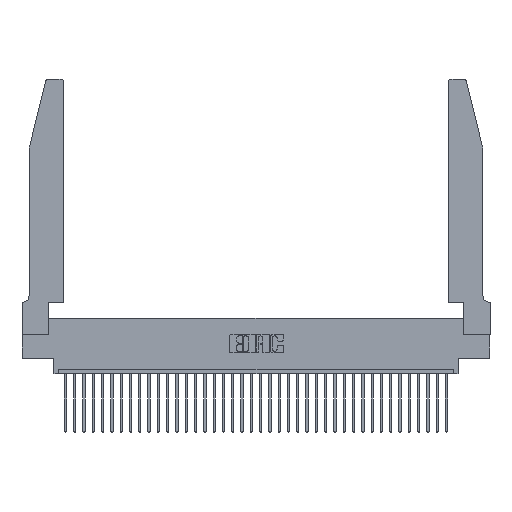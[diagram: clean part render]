
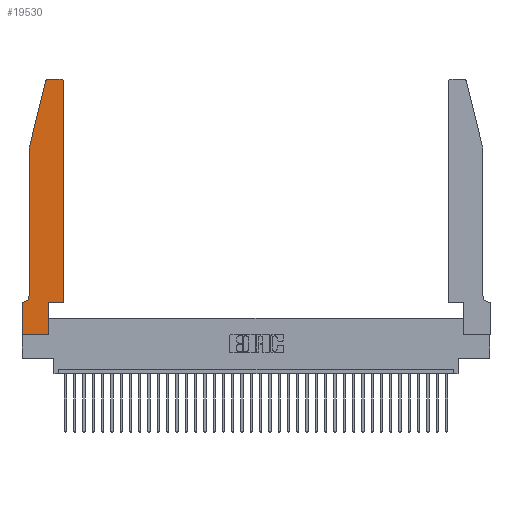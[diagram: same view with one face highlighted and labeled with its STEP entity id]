
A CAD part, top view. The second image highlights one B-rep face of the part: STEP entity #19530.
In plain terms, the highlighted planar face has unit normal (0, 0, 1).
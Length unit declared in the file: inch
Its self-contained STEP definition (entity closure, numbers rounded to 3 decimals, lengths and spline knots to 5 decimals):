
#104 = ORIENTED_EDGE ( 'NONE', *, *, #18381, .T. ) ;
#1021 = ORIENTED_EDGE ( 'NONE', *, *, #34340, .T. ) ;
#1047 = DIRECTION ( 'NONE',  ( 0., 0., 1. ) ) ;
#1149 = EDGE_CURVE ( 'NONE', #9233, #17301, #22306, .T. ) ;
#1381 = LINE ( 'NONE', #8915, #28766 ) ;
#1990 = DIRECTION ( 'NONE',  ( 0., 0., -1. ) ) ;
#2194 = DIRECTION ( 'NONE',  ( 0., -1., 0. ) ) ;
#2860 = CARTESIAN_POINT ( 'NONE',  ( 0.2865, 0.35, 0.37 ) ) ;
#3913 = CARTESIAN_POINT ( 'NONE',  ( 0.0755, 2., 0.37 ) ) ;
#4908 = ORIENTED_EDGE ( 'NONE', *, *, #8426, .T. ) ;
#5167 = CARTESIAN_POINT ( 'NONE',  ( 0.4505, 0.35, 0.37 ) ) ;
#5581 = VERTEX_POINT ( 'NONE', #16289 ) ;
#5893 = LINE ( 'NONE', #32503, #34131 ) ;
#6058 = ORIENTED_EDGE ( 'NONE', *, *, #6777, .T. ) ;
#6255 = PLANE ( 'NONE',  #33930 ) ;
#6259 = CARTESIAN_POINT ( 'NONE',  ( 0.4205, 2.75, 0.37 ) ) ;
#6381 = DIRECTION ( 'NONE',  ( 1., 0., 0. ) ) ;
#6386 = VECTOR ( 'NONE', #28680, 39.37008 ) ;
#6445 = CARTESIAN_POINT ( 'NONE',  ( 0.4505, 2.72, 0.37 ) ) ;
#6777 = EDGE_CURVE ( 'NONE', #31372, #21682, #1381, .T. ) ;
#7973 = DIRECTION ( 'NONE',  ( 0., 1., 0. ) ) ;
#8138 = CARTESIAN_POINT ( 'NONE',  ( 0.2865, 0., 0.37 ) ) ;
#8152 = FACE_OUTER_BOUND ( 'NONE', #36357, .T. ) ;
#8426 = EDGE_CURVE ( 'NONE', #9585, #5581, #9651, .T. ) ;
#8915 = CARTESIAN_POINT ( 'NONE',  ( 0.0755, 0.35, 0.37 ) ) ;
#9003 = VECTOR ( 'NONE', #2194, 39.37008 ) ;
#9174 = DIRECTION ( 'NONE',  ( -1., 0., 0. ) ) ;
#9233 = VERTEX_POINT ( 'NONE', #18907 ) ;
#9259 = ORIENTED_EDGE ( 'NONE', *, *, #11020, .T. ) ;
#9376 = DIRECTION ( 'NONE',  ( -1., 0., 0. ) ) ;
#9585 = VERTEX_POINT ( 'NONE', #6259 ) ;
#9651 = LINE ( 'NONE', #29414, #15865 ) ;
#9731 = VERTEX_POINT ( 'NONE', #2860 ) ;
#9755 = VERTEX_POINT ( 'NONE', #19752 ) ;
#10150 = DIRECTION ( 'NONE',  ( 1., 0., 0. ) ) ;
#10426 = ORIENTED_EDGE ( 'NONE', *, *, #25090, .T. ) ;
#11020 = EDGE_CURVE ( 'NONE', #18442, #15830, #34611, .T. ) ;
#11919 = DIRECTION ( 'NONE',  ( 0., 0., 1. ) ) ;
#12272 = VERTEX_POINT ( 'NONE', #26230 ) ;
#12887 = DIRECTION ( 'NONE',  ( 0., 0., 1. ) ) ;
#13012 = CARTESIAN_POINT ( 'NONE',  ( 0.4205, 2.72, 0.37 ) ) ;
#13457 = CARTESIAN_POINT ( 'NONE',  ( 0., 0., 0.37 ) ) ;
#13645 = CIRCLE ( 'NONE', #14404, 0.07 ) ;
#14021 = CARTESIAN_POINT ( 'NONE',  ( 0., 0., 0.37 ) ) ;
#14402 = CARTESIAN_POINT ( 'NONE',  ( 0., 0.35, 0.37 ) ) ;
#14404 = AXIS2_PLACEMENT_3D ( 'NONE', #25024, #1990, #27803 ) ;
#14706 = AXIS2_PLACEMENT_3D ( 'NONE', #29063, #1047, #32008 ) ;
#15378 = CARTESIAN_POINT ( 'NONE',  ( 0.0755, 0.42, 0.37 ) ) ;
#15453 = DIRECTION ( 'NONE',  ( 1., 0., 0. ) ) ;
#15830 = VERTEX_POINT ( 'NONE', #6445 ) ;
#15865 = VECTOR ( 'NONE', #9376, 39.37008 ) ;
#16289 = CARTESIAN_POINT ( 'NONE',  ( 0.284, 2.75, 0.37 ) ) ;
#16470 = VECTOR ( 'NONE', #27167, 39.37008 ) ;
#16622 = LINE ( 'NONE', #33528, #21451 ) ;
#16752 = ORIENTED_EDGE ( 'NONE', *, *, #1149, .T. ) ;
#16929 = VERTEX_POINT ( 'NONE', #8138 ) ;
#17301 = VERTEX_POINT ( 'NONE', #15378 ) ;
#18087 = EDGE_CURVE ( 'NONE', #21682, #12272, #34249, .T. ) ;
#18208 = ORIENTED_EDGE ( 'NONE', *, *, #24212, .T. ) ;
#18381 = EDGE_CURVE ( 'NONE', #5581, #9755, #33886, .T. ) ;
#18442 = VERTEX_POINT ( 'NONE', #23598 ) ;
#18907 = CARTESIAN_POINT ( 'NONE',  ( 0.0755, 2., 0.37 ) ) ;
#19153 = ORIENTED_EDGE ( 'NONE', *, *, #18087, .T. ) ;
#19207 = ORIENTED_EDGE ( 'NONE', *, *, #26116, .T. ) ;
#19271 = VECTOR ( 'NONE', #22269, 39.37008 ) ;
#19530 = ADVANCED_FACE ( 'NONE', ( #8152 ), #6255, .T. ) ;
#19752 = CARTESIAN_POINT ( 'NONE',  ( 0.25487, 2.72718, 0.37 ) ) ;
#20029 = DIRECTION ( 'NONE',  ( 0., 1., 0. ) ) ;
#20294 = CARTESIAN_POINT ( 'NONE',  ( 0., 0.35, 0.37 ) ) ;
#20967 = ORIENTED_EDGE ( 'NONE', *, *, #26812, .T. ) ;
#21368 = VECTOR ( 'NONE', #7973, 39.37008 ) ;
#21451 = VECTOR ( 'NONE', #20029, 39.37008 ) ;
#21682 = VERTEX_POINT ( 'NONE', #14402 ) ;
#21771 = LINE ( 'NONE', #13457, #16470 ) ;
#22269 = DIRECTION ( 'NONE',  ( 0., -1., 0. ) ) ;
#22306 = LINE ( 'NONE', #3913, #9003 ) ;
#23598 = CARTESIAN_POINT ( 'NONE',  ( 0.4505, 0.35, 0.37 ) ) ;
#24065 = AXIS2_PLACEMENT_3D ( 'NONE', #13012, #12887, #15453 ) ;
#24212 = EDGE_CURVE ( 'NONE', #9731, #18442, #5893, .T. ) ;
#25024 = CARTESIAN_POINT ( 'NONE',  ( 0.0055, 0.42, 0.37 ) ) ;
#25090 = EDGE_CURVE ( 'NONE', #17301, #31372, #13645, .T. ) ;
#25116 = ORIENTED_EDGE ( 'NONE', *, *, #33382, .T. ) ;
#25815 = LINE ( 'NONE', #28440, #6386 ) ;
#26116 = EDGE_CURVE ( 'NONE', #16929, #9731, #16622, .T. ) ;
#26230 = CARTESIAN_POINT ( 'NONE',  ( 0., 0., 0.37 ) ) ;
#26812 = EDGE_CURVE ( 'NONE', #9755, #9233, #25815, .T. ) ;
#27167 = DIRECTION ( 'NONE',  ( 1., 0., 0. ) ) ;
#27803 = DIRECTION ( 'NONE',  ( -1., 0., 0. ) ) ;
#28440 = CARTESIAN_POINT ( 'NONE',  ( 0.0755, 2., 0.37 ) ) ;
#28623 = CARTESIAN_POINT ( 'NONE',  ( 0.0055, 0.35, 0.37 ) ) ;
#28680 = DIRECTION ( 'NONE',  ( -0.239, -0.971, 0. ) ) ;
#28766 = VECTOR ( 'NONE', #9174, 39.37008 ) ;
#29063 = CARTESIAN_POINT ( 'NONE',  ( 0.284, 2.72, 0.37 ) ) ;
#29414 = CARTESIAN_POINT ( 'NONE',  ( 0.2605, 2.75, 0.37 ) ) ;
#31372 = VERTEX_POINT ( 'NONE', #28623 ) ;
#32008 = DIRECTION ( 'NONE',  ( 1., 0., 0. ) ) ;
#32503 = CARTESIAN_POINT ( 'NONE',  ( 0.4505, 0.35, 0.37 ) ) ;
#33382 = EDGE_CURVE ( 'NONE', #12272, #16929, #21771, .T. ) ;
#33389 = CIRCLE ( 'NONE', #24065, 0.03 ) ;
#33528 = CARTESIAN_POINT ( 'NONE',  ( 0.2865, 0.35, 0.37 ) ) ;
#33886 = CIRCLE ( 'NONE', #14706, 0.03 ) ;
#33930 = AXIS2_PLACEMENT_3D ( 'NONE', #20294, #11919, #6381 ) ;
#34131 = VECTOR ( 'NONE', #10150, 39.37008 ) ;
#34249 = LINE ( 'NONE', #14021, #19271 ) ;
#34340 = EDGE_CURVE ( 'NONE', #15830, #9585, #33389, .T. ) ;
#34611 = LINE ( 'NONE', #5167, #21368 ) ;
#36357 = EDGE_LOOP ( 'NONE', ( #4908, #104, #20967, #16752, #10426, #6058, #19153, #25116, #19207, #18208, #9259, #1021 ) ) ;
